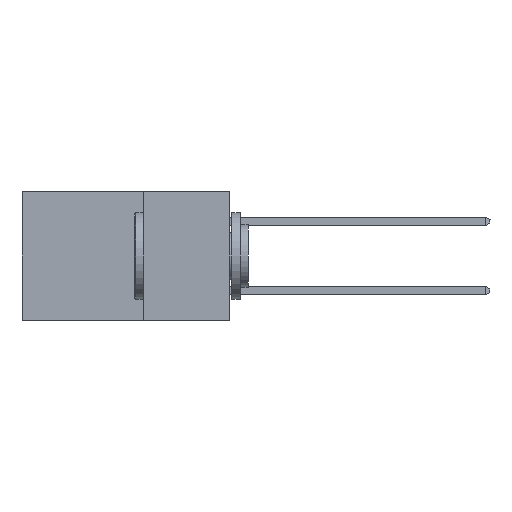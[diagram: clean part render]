
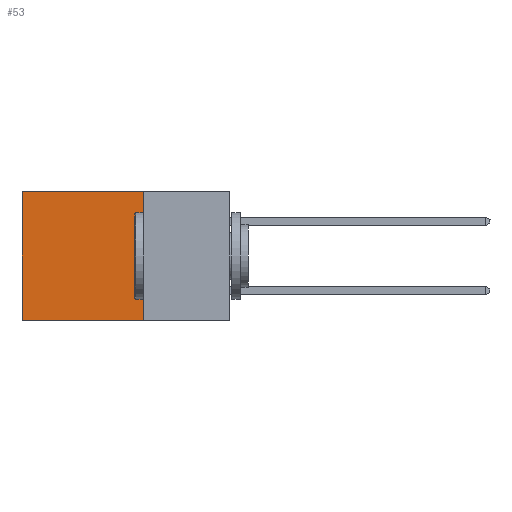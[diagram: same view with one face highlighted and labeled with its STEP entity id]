
A CAD part, left-side view. The second image highlights one B-rep face of the part: STEP entity #53.
In plain terms, the highlighted planar face has unit normal (-1, 0, 0).
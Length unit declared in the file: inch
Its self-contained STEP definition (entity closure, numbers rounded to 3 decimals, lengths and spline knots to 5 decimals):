
#53 = ADVANCED_FACE ( 'NONE', ( #8364 ), #7764, .F. ) ;
#636 = ORIENTED_EDGE ( 'NONE', *, *, #6433, .T. ) ;
#917 = EDGE_CURVE ( 'NONE', #6076, #7133, #12888, .T. ) ;
#1121 = AXIS2_PLACEMENT_3D ( 'NONE', #11342, #1973, #2026 ) ;
#1249 = LINE ( 'NONE', #2160, #8386 ) ;
#1973 = DIRECTION ( 'NONE',  ( 1., 0., 0. ) ) ;
#2026 = DIRECTION ( 'NONE',  ( 0., 0., -1. ) ) ;
#2160 = CARTESIAN_POINT ( 'NONE',  ( 0.298, 0.25, 0. ) ) ;
#2423 = ORIENTED_EDGE ( 'NONE', *, *, #917, .F. ) ;
#2803 = ORIENTED_EDGE ( 'NONE', *, *, #13701, .F. ) ;
#3116 = VECTOR ( 'NONE', #9588, 39.37008 ) ;
#3183 = CARTESIAN_POINT ( 'NONE',  ( 0.298, 0.6, 0. ) ) ;
#3646 = VERTEX_POINT ( 'NONE', #3183 ) ;
#4975 = CARTESIAN_POINT ( 'NONE',  ( 0.298, 0.6, 0. ) ) ;
#6076 = VERTEX_POINT ( 'NONE', #10165 ) ;
#6195 = VERTEX_POINT ( 'NONE', #14041 ) ;
#6212 = EDGE_LOOP ( 'NONE', ( #636, #2423, #2803, #6411 ) ) ;
#6411 = ORIENTED_EDGE ( 'NONE', *, *, #9118, .T. ) ;
#6433 = EDGE_CURVE ( 'NONE', #3646, #7133, #6954, .T. ) ;
#6940 = DIRECTION ( 'NONE',  ( 0., 1., 0. ) ) ;
#6954 = LINE ( 'NONE', #4975, #14259 ) ;
#7133 = VERTEX_POINT ( 'NONE', #7146 ) ;
#7146 = CARTESIAN_POINT ( 'NONE',  ( 0.298, 0.6, -0.37 ) ) ;
#7665 = DIRECTION ( 'NONE',  ( 0., 1., 0. ) ) ;
#7764 = PLANE ( 'NONE',  #1121 ) ;
#8364 = FACE_OUTER_BOUND ( 'NONE', #6212, .T. ) ;
#8386 = VECTOR ( 'NONE', #6940, 39.37008 ) ;
#9118 = EDGE_CURVE ( 'NONE', #6195, #3646, #1249, .T. ) ;
#9588 = DIRECTION ( 'NONE',  ( 0., 0., -1. ) ) ;
#10165 = CARTESIAN_POINT ( 'NONE',  ( 0.298, 0.25, -0.37 ) ) ;
#11342 = CARTESIAN_POINT ( 'NONE',  ( 0.298, 0.25, 0. ) ) ;
#11771 = VECTOR ( 'NONE', #7665, 39.37008 ) ;
#11862 = LINE ( 'NONE', #14309, #3116 ) ;
#12425 = CARTESIAN_POINT ( 'NONE',  ( 0.298, 0.25, -0.37 ) ) ;
#12888 = LINE ( 'NONE', #12425, #11771 ) ;
#13133 = DIRECTION ( 'NONE',  ( 0., 0., -1. ) ) ;
#13701 = EDGE_CURVE ( 'NONE', #6195, #6076, #11862, .T. ) ;
#14041 = CARTESIAN_POINT ( 'NONE',  ( 0.298, 0.25, 0. ) ) ;
#14259 = VECTOR ( 'NONE', #13133, 39.37008 ) ;
#14309 = CARTESIAN_POINT ( 'NONE',  ( 0.298, 0.25, 0. ) ) ;
